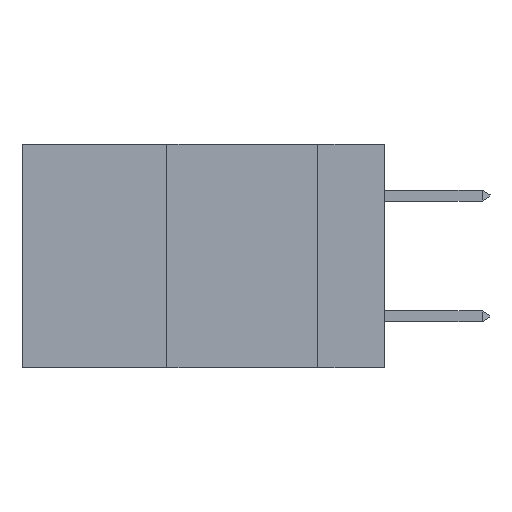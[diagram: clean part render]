
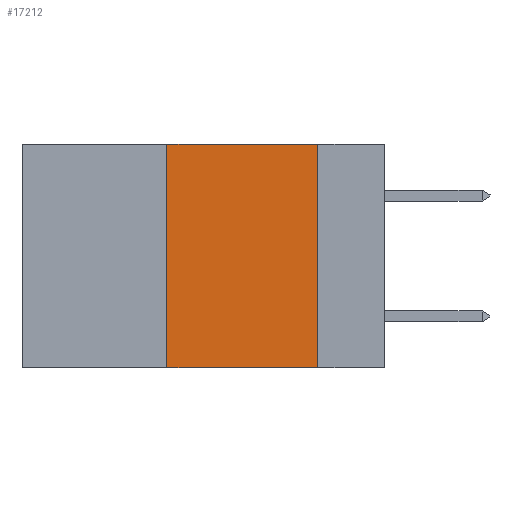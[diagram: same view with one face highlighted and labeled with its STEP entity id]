
A CAD part, left-side view. The second image highlights one B-rep face of the part: STEP entity #17212.
In plain terms, the highlighted planar face has unit normal (-1, 0, 0).
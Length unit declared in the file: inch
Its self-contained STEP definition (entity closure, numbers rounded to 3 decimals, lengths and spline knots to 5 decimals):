
#595 = DIRECTION ( 'NONE',  ( 0., 0., -1. ) ) ;
#611 = VERTEX_POINT ( 'NONE', #4963 ) ;
#663 = LINE ( 'NONE', #3370, #18060 ) ;
#740 = EDGE_LOOP ( 'NONE', ( #3723, #11045, #17131, #14915 ) ) ;
#904 = CARTESIAN_POINT ( 'NONE',  ( 0., 0.11, 0. ) ) ;
#2930 = VECTOR ( 'NONE', #6207, 39.37008 ) ;
#3306 = DIRECTION ( 'NONE',  ( 1., 0., 0. ) ) ;
#3370 = CARTESIAN_POINT ( 'NONE',  ( 0., 0.6, -0.37 ) ) ;
#3723 = ORIENTED_EDGE ( 'NONE', *, *, #8284, .F. ) ;
#4963 = CARTESIAN_POINT ( 'NONE',  ( 0., 0.36, -0.37 ) ) ;
#5283 = VERTEX_POINT ( 'NONE', #14450 ) ;
#5885 = VERTEX_POINT ( 'NONE', #7570 ) ;
#5914 = PLANE ( 'NONE',  #15997 ) ;
#6207 = DIRECTION ( 'NONE',  ( 0., 0., 1. ) ) ;
#6235 = CARTESIAN_POINT ( 'NONE',  ( 0., 0.6, 0. ) ) ;
#6580 = CARTESIAN_POINT ( 'NONE',  ( 0., 0.36, 0. ) ) ;
#6856 = VECTOR ( 'NONE', #13851, 39.37008 ) ;
#6982 = VERTEX_POINT ( 'NONE', #15584 ) ;
#7180 = FACE_OUTER_BOUND ( 'NONE', #740, .T. ) ;
#7456 = EDGE_CURVE ( 'NONE', #611, #6982, #663, .T. ) ;
#7527 = DIRECTION ( 'NONE',  ( 0., -1., 0. ) ) ;
#7570 = CARTESIAN_POINT ( 'NONE',  ( 0., 0.11, 0. ) ) ;
#8168 = DIRECTION ( 'NONE',  ( 0., -1., 0. ) ) ;
#8284 = EDGE_CURVE ( 'NONE', #5885, #6982, #12786, .T. ) ;
#9787 = EDGE_CURVE ( 'NONE', #5283, #5885, #16408, .T. ) ;
#10793 = EDGE_CURVE ( 'NONE', #611, #5283, #11571, .T. ) ;
#11045 = ORIENTED_EDGE ( 'NONE', *, *, #9787, .F. ) ;
#11571 = LINE ( 'NONE', #6580, #2930 ) ;
#12685 = VECTOR ( 'NONE', #8168, 39.37008 ) ;
#12786 = LINE ( 'NONE', #904, #6856 ) ;
#13783 = CARTESIAN_POINT ( 'NONE',  ( 0., 0.6, 0. ) ) ;
#13851 = DIRECTION ( 'NONE',  ( 0., 0., -1. ) ) ;
#14450 = CARTESIAN_POINT ( 'NONE',  ( 0., 0.36, 0. ) ) ;
#14915 = ORIENTED_EDGE ( 'NONE', *, *, #7456, .T. ) ;
#15584 = CARTESIAN_POINT ( 'NONE',  ( 0., 0.11, -0.37 ) ) ;
#15997 = AXIS2_PLACEMENT_3D ( 'NONE', #6235, #3306, #595 ) ;
#16408 = LINE ( 'NONE', #13783, #12685 ) ;
#17131 = ORIENTED_EDGE ( 'NONE', *, *, #10793, .F. ) ;
#17212 = ADVANCED_FACE ( 'NONE', ( #7180 ), #5914, .F. ) ;
#18060 = VECTOR ( 'NONE', #7527, 39.37008 ) ;
